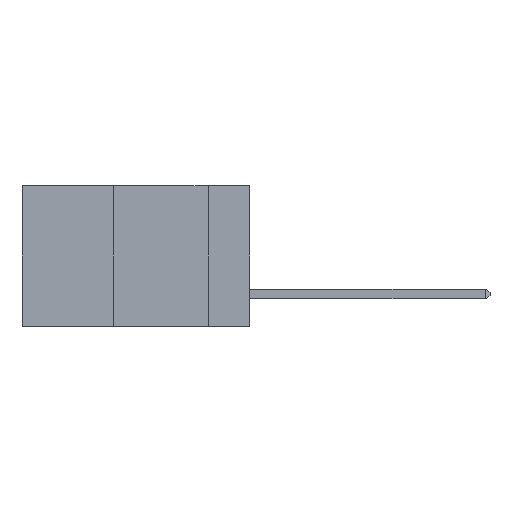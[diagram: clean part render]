
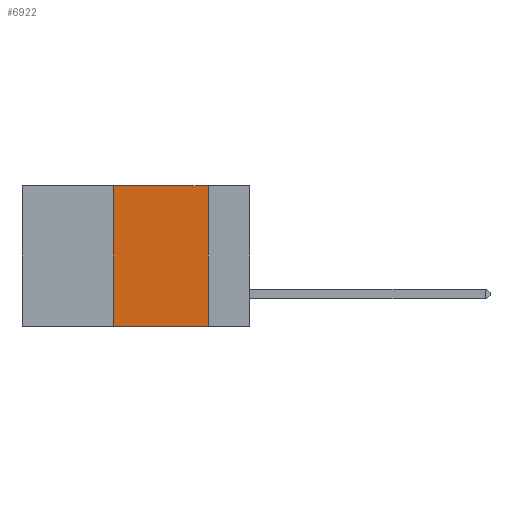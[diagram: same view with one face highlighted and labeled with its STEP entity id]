
A CAD part, left-side view. The second image highlights one B-rep face of the part: STEP entity #6922.
In plain terms, the highlighted planar face has unit normal (-1, 0, 0).
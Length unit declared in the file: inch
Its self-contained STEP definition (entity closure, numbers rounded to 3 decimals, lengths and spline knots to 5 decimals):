
#477 = CARTESIAN_POINT ( 'NONE',  ( 0., 0.6, 0. ) ) ;
#751 = ORIENTED_EDGE ( 'NONE', *, *, #24578, .F. ) ;
#1123 = CARTESIAN_POINT ( 'NONE',  ( 0., 0.11, -0.37 ) ) ;
#2115 = EDGE_CURVE ( 'NONE', #16029, #6693, #30196, .T. ) ;
#2539 = VECTOR ( 'NONE', #24376, 39.37008 ) ;
#3271 = CARTESIAN_POINT ( 'NONE',  ( 0., 0.36, 0. ) ) ;
#6063 = DIRECTION ( 'NONE',  ( 0., -1., 0. ) ) ;
#6693 = VERTEX_POINT ( 'NONE', #13253 ) ;
#6922 = ADVANCED_FACE ( 'NONE', ( #16968 ), #25957, .F. ) ;
#7428 = LINE ( 'NONE', #10616, #20828 ) ;
#7694 = CARTESIAN_POINT ( 'NONE',  ( 0., 0.6, -0.37 ) ) ;
#8867 = LINE ( 'NONE', #30211, #28632 ) ;
#9978 = EDGE_LOOP ( 'NONE', ( #751, #12987, #24853, #24129 ) ) ;
#10616 = CARTESIAN_POINT ( 'NONE',  ( 0., 0.11, 0. ) ) ;
#10851 = VERTEX_POINT ( 'NONE', #1123 ) ;
#11242 = AXIS2_PLACEMENT_3D ( 'NONE', #25861, #28397, #14165 ) ;
#11249 = VECTOR ( 'NONE', #6063, 39.37008 ) ;
#12987 = ORIENTED_EDGE ( 'NONE', *, *, #2115, .F. ) ;
#13253 = CARTESIAN_POINT ( 'NONE',  ( 0., 0.11, 0. ) ) ;
#14165 = DIRECTION ( 'NONE',  ( 0., 0., -1. ) ) ;
#15978 = DIRECTION ( 'NONE',  ( 0., 0., 1. ) ) ;
#16029 = VERTEX_POINT ( 'NONE', #3271 ) ;
#16968 = FACE_OUTER_BOUND ( 'NONE', #9978, .T. ) ;
#17169 = CARTESIAN_POINT ( 'NONE',  ( 0., 0.36, -0.37 ) ) ;
#20828 = VECTOR ( 'NONE', #22467, 39.37008 ) ;
#20912 = LINE ( 'NONE', #7694, #2539 ) ;
#22176 = EDGE_CURVE ( 'NONE', #30629, #10851, #20912, .T. ) ;
#22467 = DIRECTION ( 'NONE',  ( 0., 0., -1. ) ) ;
#24129 = ORIENTED_EDGE ( 'NONE', *, *, #22176, .T. ) ;
#24376 = DIRECTION ( 'NONE',  ( 0., -1., 0. ) ) ;
#24578 = EDGE_CURVE ( 'NONE', #6693, #10851, #7428, .T. ) ;
#24853 = ORIENTED_EDGE ( 'NONE', *, *, #25343, .F. ) ;
#25343 = EDGE_CURVE ( 'NONE', #30629, #16029, #8867, .T. ) ;
#25861 = CARTESIAN_POINT ( 'NONE',  ( 0., 0.6, 0. ) ) ;
#25957 = PLANE ( 'NONE',  #11242 ) ;
#28397 = DIRECTION ( 'NONE',  ( 1., 0., 0. ) ) ;
#28632 = VECTOR ( 'NONE', #15978, 39.37008 ) ;
#30196 = LINE ( 'NONE', #477, #11249 ) ;
#30211 = CARTESIAN_POINT ( 'NONE',  ( 0., 0.36, 0. ) ) ;
#30629 = VERTEX_POINT ( 'NONE', #17169 ) ;
